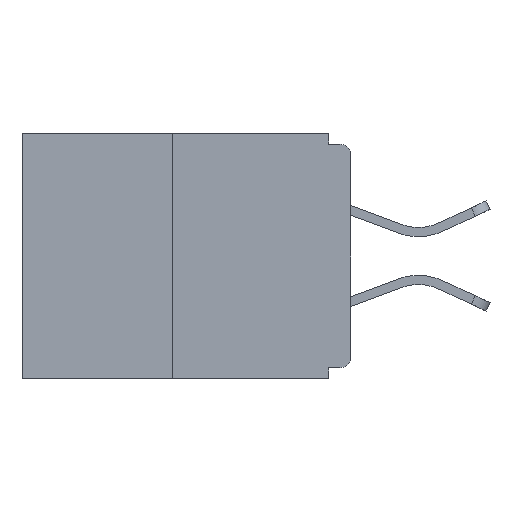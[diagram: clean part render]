
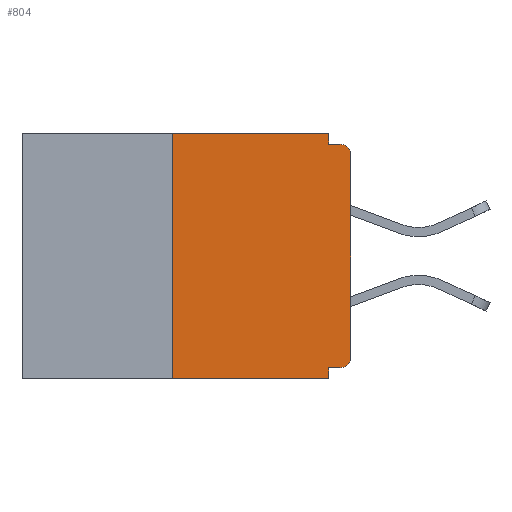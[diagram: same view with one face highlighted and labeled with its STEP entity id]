
A CAD part, left-side view. The second image highlights one B-rep face of the part: STEP entity #804.
In plain terms, the highlighted planar face has unit normal (-1, 0, 0).
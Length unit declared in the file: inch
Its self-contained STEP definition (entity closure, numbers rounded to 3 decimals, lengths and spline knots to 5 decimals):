
#586 = CARTESIAN_POINT ( 'NONE',  ( 0., 0.015, -0.015 ) ) ;
#675 = AXIS2_PLACEMENT_3D ( 'NONE', #6457, #14069, #6291 ) ;
#804 = ADVANCED_FACE ( 'NONE', ( #11521 ), #6319, .F. ) ;
#888 = CARTESIAN_POINT ( 'NONE',  ( 0., 0.25, 0. ) ) ;
#1062 = VERTEX_POINT ( 'NONE', #10538 ) ;
#1106 = DIRECTION ( 'NONE',  ( 0., 0., 1. ) ) ;
#1193 = CARTESIAN_POINT ( 'NONE',  ( 0., 0., -0.03 ) ) ;
#1199 = ORIENTED_EDGE ( 'NONE', *, *, #1224, .T. ) ;
#1224 = EDGE_CURVE ( 'NONE', #11413, #4442, #3452, .T. ) ;
#1334 = CARTESIAN_POINT ( 'NONE',  ( 0., 0.015, -0.328 ) ) ;
#1378 = EDGE_CURVE ( 'NONE', #6715, #4940, #1392, .T. ) ;
#1392 = LINE ( 'NONE', #8564, #6141 ) ;
#1753 = CARTESIAN_POINT ( 'NONE',  ( 0., 0.031, 0. ) ) ;
#2653 = CARTESIAN_POINT ( 'NONE',  ( 0., 0., -0.015 ) ) ;
#2807 = CARTESIAN_POINT ( 'NONE',  ( 0., 0.015, -0.03 ) ) ;
#2814 = CARTESIAN_POINT ( 'NONE',  ( 0., 0.031, -0.328 ) ) ;
#3400 = DIRECTION ( 'NONE',  ( 0., 1., 0. ) ) ;
#3452 = LINE ( 'NONE', #8371, #11166 ) ;
#3661 = CARTESIAN_POINT ( 'NONE',  ( 0., 0.25, -0.343 ) ) ;
#3898 = DIRECTION ( 'NONE',  ( 1., 0., 0. ) ) ;
#4016 = LINE ( 'NONE', #2653, #13298 ) ;
#4066 = ORIENTED_EDGE ( 'NONE', *, *, #12160, .F. ) ;
#4107 = EDGE_CURVE ( 'NONE', #9382, #13562, #4016, .T. ) ;
#4442 = VERTEX_POINT ( 'NONE', #13504 ) ;
#4748 = DIRECTION ( 'NONE',  ( 0., -1., 0. ) ) ;
#4936 = DIRECTION ( 'NONE',  ( 0., -1., 0. ) ) ;
#4940 = VERTEX_POINT ( 'NONE', #14151 ) ;
#5062 = ORIENTED_EDGE ( 'NONE', *, *, #12452, .T. ) ;
#5128 = ORIENTED_EDGE ( 'NONE', *, *, #9059, .F. ) ;
#5131 = LINE ( 'NONE', #12290, #8384 ) ;
#5331 = VERTEX_POINT ( 'NONE', #2814 ) ;
#5447 = CIRCLE ( 'NONE', #9706, 0.015 ) ;
#6065 = DIRECTION ( 'NONE',  ( 0., 0., -1. ) ) ;
#6141 = VECTOR ( 'NONE', #9629, 39.37008 ) ;
#6258 = ORIENTED_EDGE ( 'NONE', *, *, #6656, .T. ) ;
#6291 = DIRECTION ( 'NONE',  ( 0., 0., -1. ) ) ;
#6319 = PLANE ( 'NONE',  #13353 ) ;
#6457 = CARTESIAN_POINT ( 'NONE',  ( 0., 0.015, -0.313 ) ) ;
#6630 = EDGE_LOOP ( 'NONE', ( #9716, #7450, #1199, #5128, #4066, #9125, #5062, #6258, #7961, #7766 ) ) ;
#6656 = EDGE_CURVE ( 'NONE', #7999, #13562, #5447, .T. ) ;
#6715 = VERTEX_POINT ( 'NONE', #888 ) ;
#6939 = VECTOR ( 'NONE', #12267, 39.37008 ) ;
#7103 = VECTOR ( 'NONE', #7325, 39.37008 ) ;
#7325 = DIRECTION ( 'NONE',  ( 0., 0., -1. ) ) ;
#7450 = ORIENTED_EDGE ( 'NONE', *, *, #10383, .F. ) ;
#7567 = VECTOR ( 'NONE', #1106, 39.37008 ) ;
#7632 = LINE ( 'NONE', #1753, #7103 ) ;
#7766 = ORIENTED_EDGE ( 'NONE', *, *, #8953, .F. ) ;
#7961 = ORIENTED_EDGE ( 'NONE', *, *, #4107, .F. ) ;
#7999 = VERTEX_POINT ( 'NONE', #1193 ) ;
#8059 = VERTEX_POINT ( 'NONE', #1334 ) ;
#8371 = CARTESIAN_POINT ( 'NONE',  ( 0., 0.46, -0.343 ) ) ;
#8384 = VECTOR ( 'NONE', #11337, 39.37008 ) ;
#8564 = CARTESIAN_POINT ( 'NONE',  ( 0., 0.46, 0. ) ) ;
#8677 = CARTESIAN_POINT ( 'NONE',  ( 0., 0.46, 0. ) ) ;
#8842 = CARTESIAN_POINT ( 'NONE',  ( 0., 0.031, -0.343 ) ) ;
#8877 = CARTESIAN_POINT ( 'NONE',  ( 0., 0.25, 0. ) ) ;
#8953 = EDGE_CURVE ( 'NONE', #4940, #9382, #7632, .T. ) ;
#9059 = EDGE_CURVE ( 'NONE', #5331, #4442, #9874, .T. ) ;
#9125 = ORIENTED_EDGE ( 'NONE', *, *, #10235, .T. ) ;
#9274 = VECTOR ( 'NONE', #3400, 39.37008 ) ;
#9382 = VERTEX_POINT ( 'NONE', #12122 ) ;
#9629 = DIRECTION ( 'NONE',  ( 0., -1., 0. ) ) ;
#9706 = AXIS2_PLACEMENT_3D ( 'NONE', #2807, #12619, #6065 ) ;
#9716 = ORIENTED_EDGE ( 'NONE', *, *, #1378, .F. ) ;
#9808 = CARTESIAN_POINT ( 'NONE',  ( 0., 0., -0.328 ) ) ;
#9817 = LINE ( 'NONE', #8877, #7567 ) ;
#9874 = LINE ( 'NONE', #8842, #6939 ) ;
#10235 = EDGE_CURVE ( 'NONE', #8059, #1062, #12415, .T. ) ;
#10383 = EDGE_CURVE ( 'NONE', #11413, #6715, #9817, .T. ) ;
#10482 = DIRECTION ( 'NONE',  ( 0., 0., -1. ) ) ;
#10538 = CARTESIAN_POINT ( 'NONE',  ( 0., 0., -0.313 ) ) ;
#11166 = VECTOR ( 'NONE', #4936, 39.37008 ) ;
#11337 = DIRECTION ( 'NONE',  ( 0., 0., 1. ) ) ;
#11413 = VERTEX_POINT ( 'NONE', #3661 ) ;
#11521 = FACE_OUTER_BOUND ( 'NONE', #6630, .T. ) ;
#12122 = CARTESIAN_POINT ( 'NONE',  ( 0., 0.031, -0.015 ) ) ;
#12160 = EDGE_CURVE ( 'NONE', #8059, #5331, #12199, .T. ) ;
#12199 = LINE ( 'NONE', #9808, #9274 ) ;
#12267 = DIRECTION ( 'NONE',  ( 0., 0., -1. ) ) ;
#12290 = CARTESIAN_POINT ( 'NONE',  ( 0., 0., 0. ) ) ;
#12415 = CIRCLE ( 'NONE', #675, 0.015 ) ;
#12452 = EDGE_CURVE ( 'NONE', #1062, #7999, #5131, .T. ) ;
#12619 = DIRECTION ( 'NONE',  ( -1., 0., 0. ) ) ;
#13298 = VECTOR ( 'NONE', #4748, 39.37008 ) ;
#13353 = AXIS2_PLACEMENT_3D ( 'NONE', #8677, #3898, #10482 ) ;
#13504 = CARTESIAN_POINT ( 'NONE',  ( 0., 0.031, -0.343 ) ) ;
#13562 = VERTEX_POINT ( 'NONE', #586 ) ;
#14069 = DIRECTION ( 'NONE',  ( -1., 0., 0. ) ) ;
#14151 = CARTESIAN_POINT ( 'NONE',  ( 0., 0.031, 0. ) ) ;
